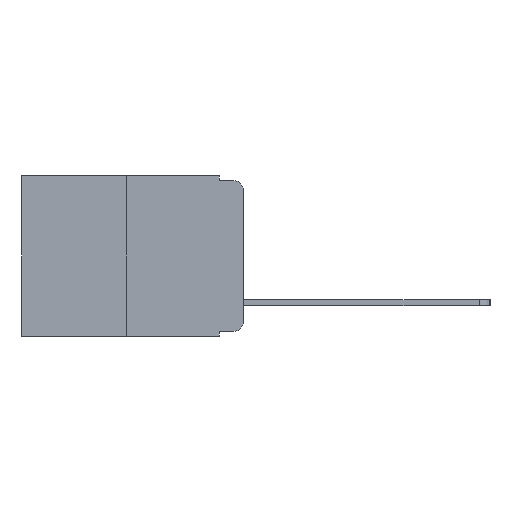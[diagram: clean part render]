
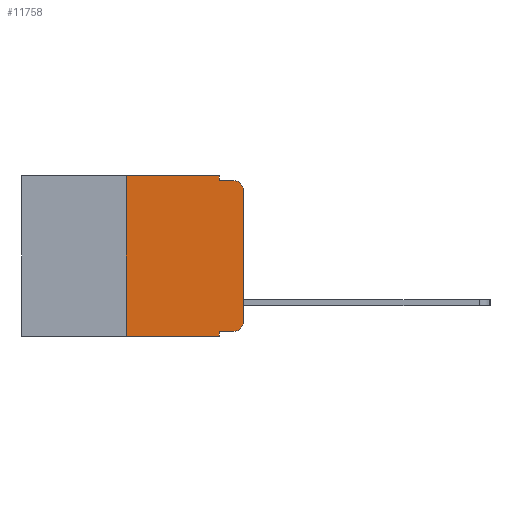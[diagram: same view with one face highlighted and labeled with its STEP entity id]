
A CAD part, left-side view. The second image highlights one B-rep face of the part: STEP entity #11758.
In plain terms, the highlighted planar face has unit normal (-1, 0, 0).
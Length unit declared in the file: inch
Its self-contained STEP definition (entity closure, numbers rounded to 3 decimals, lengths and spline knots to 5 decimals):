
#179 = EDGE_CURVE ( 'NONE', #8561, #3623, #12340, .T. ) ;
#202 = PLANE ( 'NONE',  #3186 ) ;
#313 = DIRECTION ( 'NONE',  ( 0., 0., -1. ) ) ;
#448 = FACE_OUTER_BOUND ( 'NONE', #11480, .T. ) ;
#490 = ORIENTED_EDGE ( 'NONE', *, *, #13386, .F. ) ;
#560 = ORIENTED_EDGE ( 'NONE', *, *, #13745, .T. ) ;
#622 = CARTESIAN_POINT ( 'NONE',  ( 0., 0.051, 0. ) ) ;
#681 = DIRECTION ( 'NONE',  ( -1., 0., 0. ) ) ;
#696 = VERTEX_POINT ( 'NONE', #7370 ) ;
#796 = DIRECTION ( 'NONE',  ( 0., 0., 1. ) ) ;
#812 = EDGE_CURVE ( 'NONE', #1642, #9123, #7688, .T. ) ;
#841 = ORIENTED_EDGE ( 'NONE', *, *, #1226, .T. ) ;
#1029 = ORIENTED_EDGE ( 'NONE', *, *, #9497, .F. ) ;
#1165 = DIRECTION ( 'NONE',  ( 0., -1., 0. ) ) ;
#1178 = CARTESIAN_POINT ( 'NONE',  ( 0., 0.051, -0.333 ) ) ;
#1226 = EDGE_CURVE ( 'NONE', #4723, #4150, #5395, .T. ) ;
#1228 = EDGE_CURVE ( 'NONE', #2133, #696, #8401, .T. ) ;
#1250 = EDGE_CURVE ( 'NONE', #5847, #696, #13618, .T. ) ;
#1642 = VERTEX_POINT ( 'NONE', #1178 ) ;
#1696 = EDGE_CURVE ( 'NONE', #9123, #7210, #8385, .T. ) ;
#1755 = LINE ( 'NONE', #6153, #12697 ) ;
#1774 = DIRECTION ( 'NONE',  ( 0., 0., -1. ) ) ;
#1847 = CARTESIAN_POINT ( 'NONE',  ( 0., 0.02, -0.03 ) ) ;
#2133 = VERTEX_POINT ( 'NONE', #3835 ) ;
#2296 = ORIENTED_EDGE ( 'NONE', *, *, #179, .F. ) ;
#2415 = CARTESIAN_POINT ( 'NONE',  ( 0., 0., 0. ) ) ;
#2421 = VECTOR ( 'NONE', #1165, 39.37008 ) ;
#2504 = CARTESIAN_POINT ( 'NONE',  ( 0., 0.473, 0. ) ) ;
#2552 = DIRECTION ( 'NONE',  ( 1., 0., 0. ) ) ;
#2857 = AXIS2_PLACEMENT_3D ( 'NONE', #1847, #681, #313 ) ;
#3186 = AXIS2_PLACEMENT_3D ( 'NONE', #2504, #2552, #10299 ) ;
#3623 = VERTEX_POINT ( 'NONE', #12180 ) ;
#3835 = CARTESIAN_POINT ( 'NONE',  ( 0., 0.051, -0.01 ) ) ;
#4150 = VERTEX_POINT ( 'NONE', #4305 ) ;
#4254 = VECTOR ( 'NONE', #11246, 39.37008 ) ;
#4305 = CARTESIAN_POINT ( 'NONE',  ( 0., 0.051, -0.343 ) ) ;
#4393 = ORIENTED_EDGE ( 'NONE', *, *, #10250, .F. ) ;
#4701 = VECTOR ( 'NONE', #8603, 39.37008 ) ;
#4723 = VERTEX_POINT ( 'NONE', #12750 ) ;
#5315 = CARTESIAN_POINT ( 'NONE',  ( 0., 0., -0.313 ) ) ;
#5395 = LINE ( 'NONE', #11256, #2421 ) ;
#5485 = CARTESIAN_POINT ( 'NONE',  ( 0., 0.02, -0.313 ) ) ;
#5487 = CARTESIAN_POINT ( 'NONE',  ( 0., 0.02, -0.333 ) ) ;
#5617 = ORIENTED_EDGE ( 'NONE', *, *, #1228, .F. ) ;
#5785 = DIRECTION ( 'NONE',  ( -1., 0., 0. ) ) ;
#5847 = VERTEX_POINT ( 'NONE', #6098 ) ;
#6098 = CARTESIAN_POINT ( 'NONE',  ( 0., 0., -0.03 ) ) ;
#6153 = CARTESIAN_POINT ( 'NONE',  ( 0., 0.051, 0. ) ) ;
#6519 = LINE ( 'NONE', #622, #11931 ) ;
#7210 = VERTEX_POINT ( 'NONE', #5315 ) ;
#7269 = DIRECTION ( 'NONE',  ( 0., 0., -1. ) ) ;
#7324 = CARTESIAN_POINT ( 'NONE',  ( 0., 0.051, -0.333 ) ) ;
#7370 = CARTESIAN_POINT ( 'NONE',  ( 0., 0.02, -0.01 ) ) ;
#7688 = LINE ( 'NONE', #7324, #4701 ) ;
#7827 = AXIS2_PLACEMENT_3D ( 'NONE', #5485, #5785, #8015 ) ;
#8015 = DIRECTION ( 'NONE',  ( 0., 0., -1. ) ) ;
#8055 = DIRECTION ( 'NONE',  ( 0., -1., 0. ) ) ;
#8238 = ORIENTED_EDGE ( 'NONE', *, *, #1250, .T. ) ;
#8385 = CIRCLE ( 'NONE', #7827, 0.02 ) ;
#8401 = LINE ( 'NONE', #13068, #13945 ) ;
#8460 = LINE ( 'NONE', #10737, #13677 ) ;
#8561 = VERTEX_POINT ( 'NONE', #13134 ) ;
#8603 = DIRECTION ( 'NONE',  ( 0., -1., 0. ) ) ;
#9123 = VERTEX_POINT ( 'NONE', #5487 ) ;
#9497 = EDGE_CURVE ( 'NONE', #4723, #8561, #8460, .T. ) ;
#9574 = VECTOR ( 'NONE', #8055, 39.37008 ) ;
#10134 = LINE ( 'NONE', #2415, #4254 ) ;
#10250 = EDGE_CURVE ( 'NONE', #3623, #2133, #1755, .T. ) ;
#10299 = DIRECTION ( 'NONE',  ( 0., 0., -1. ) ) ;
#10633 = CARTESIAN_POINT ( 'NONE',  ( 0., 0.473, 0. ) ) ;
#10737 = CARTESIAN_POINT ( 'NONE',  ( 0., 0.25, 0. ) ) ;
#11246 = DIRECTION ( 'NONE',  ( 0., 0., 1. ) ) ;
#11256 = CARTESIAN_POINT ( 'NONE',  ( 0., 0.473, -0.343 ) ) ;
#11480 = EDGE_LOOP ( 'NONE', ( #560, #8238, #5617, #4393, #2296, #1029, #841, #490, #11550, #12026 ) ) ;
#11550 = ORIENTED_EDGE ( 'NONE', *, *, #812, .T. ) ;
#11758 = ADVANCED_FACE ( 'NONE', ( #448 ), #202, .F. ) ;
#11931 = VECTOR ( 'NONE', #1774, 39.37008 ) ;
#12026 = ORIENTED_EDGE ( 'NONE', *, *, #1696, .T. ) ;
#12180 = CARTESIAN_POINT ( 'NONE',  ( 0., 0.051, 0. ) ) ;
#12340 = LINE ( 'NONE', #10633, #9574 ) ;
#12697 = VECTOR ( 'NONE', #7269, 39.37008 ) ;
#12750 = CARTESIAN_POINT ( 'NONE',  ( 0., 0.25, -0.343 ) ) ;
#12895 = DIRECTION ( 'NONE',  ( 0., -1., 0. ) ) ;
#13068 = CARTESIAN_POINT ( 'NONE',  ( 0., 0.051, -0.01 ) ) ;
#13134 = CARTESIAN_POINT ( 'NONE',  ( 0., 0.25, 0. ) ) ;
#13386 = EDGE_CURVE ( 'NONE', #1642, #4150, #6519, .T. ) ;
#13618 = CIRCLE ( 'NONE', #2857, 0.02 ) ;
#13677 = VECTOR ( 'NONE', #796, 39.37008 ) ;
#13745 = EDGE_CURVE ( 'NONE', #7210, #5847, #10134, .T. ) ;
#13945 = VECTOR ( 'NONE', #12895, 39.37008 ) ;
